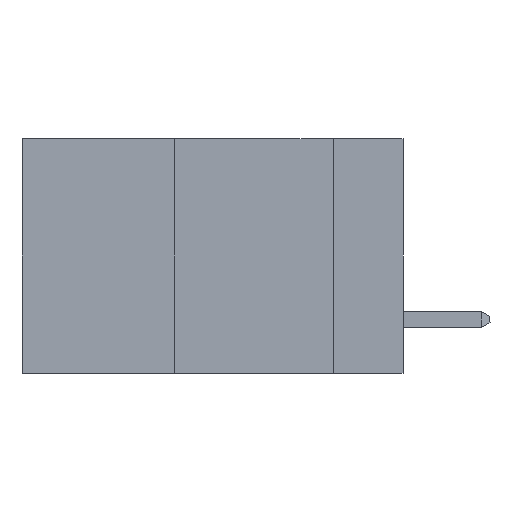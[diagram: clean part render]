
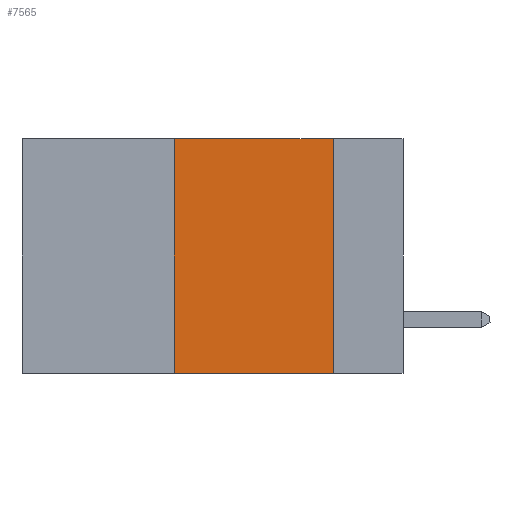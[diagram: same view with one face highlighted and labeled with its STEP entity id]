
A CAD part, left-side view. The second image highlights one B-rep face of the part: STEP entity #7565.
In plain terms, the highlighted planar face has unit normal (-1, 0, 0).
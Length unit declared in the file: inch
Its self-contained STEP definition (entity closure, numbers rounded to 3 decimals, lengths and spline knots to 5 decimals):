
#981 = VECTOR ( 'NONE', #9468, 39.37008 ) ;
#1636 = CARTESIAN_POINT ( 'NONE',  ( 0., 0.6, -0.37 ) ) ;
#1899 = CARTESIAN_POINT ( 'NONE',  ( 0., 0.36, 0. ) ) ;
#2527 = ORIENTED_EDGE ( 'NONE', *, *, #8958, .F. ) ;
#2906 = ORIENTED_EDGE ( 'NONE', *, *, #12449, .T. ) ;
#2966 = VECTOR ( 'NONE', #4611, 39.37008 ) ;
#3118 = DIRECTION ( 'NONE',  ( 0., 0., 1. ) ) ;
#3429 = LINE ( 'NONE', #1636, #981 ) ;
#3470 = CARTESIAN_POINT ( 'NONE',  ( 0., 0.6, 0. ) ) ;
#3562 = VECTOR ( 'NONE', #9497, 39.37008 ) ;
#3888 = CARTESIAN_POINT ( 'NONE',  ( 0., 0.11, 0. ) ) ;
#4048 = EDGE_CURVE ( 'NONE', #14142, #12676, #5926, .T. ) ;
#4592 = DIRECTION ( 'NONE',  ( 0., 0., -1. ) ) ;
#4611 = DIRECTION ( 'NONE',  ( 0., 0., -1. ) ) ;
#5926 = LINE ( 'NONE', #12236, #2966 ) ;
#7234 = LINE ( 'NONE', #9724, #10113 ) ;
#7475 = EDGE_LOOP ( 'NONE', ( #13849, #2527, #14164, #2906 ) ) ;
#7565 = ADVANCED_FACE ( 'NONE', ( #10115 ), #13234, .F. ) ;
#8765 = CARTESIAN_POINT ( 'NONE',  ( 0., 0.36, -0.37 ) ) ;
#8775 = CARTESIAN_POINT ( 'NONE',  ( 0., 0.11, -0.37 ) ) ;
#8958 = EDGE_CURVE ( 'NONE', #10308, #14142, #9435, .T. ) ;
#9435 = LINE ( 'NONE', #12687, #3562 ) ;
#9468 = DIRECTION ( 'NONE',  ( 0., -1., 0. ) ) ;
#9497 = DIRECTION ( 'NONE',  ( 0., -1., 0. ) ) ;
#9724 = CARTESIAN_POINT ( 'NONE',  ( 0., 0.36, 0. ) ) ;
#10113 = VECTOR ( 'NONE', #3118, 39.37008 ) ;
#10115 = FACE_OUTER_BOUND ( 'NONE', #7475, .T. ) ;
#10308 = VERTEX_POINT ( 'NONE', #1899 ) ;
#11118 = DIRECTION ( 'NONE',  ( 1., 0., 0. ) ) ;
#12236 = CARTESIAN_POINT ( 'NONE',  ( 0., 0.11, 0. ) ) ;
#12449 = EDGE_CURVE ( 'NONE', #13183, #12676, #3429, .T. ) ;
#12577 = EDGE_CURVE ( 'NONE', #13183, #10308, #7234, .T. ) ;
#12676 = VERTEX_POINT ( 'NONE', #8775 ) ;
#12687 = CARTESIAN_POINT ( 'NONE',  ( 0., 0.6, 0. ) ) ;
#13183 = VERTEX_POINT ( 'NONE', #8765 ) ;
#13234 = PLANE ( 'NONE',  #13248 ) ;
#13248 = AXIS2_PLACEMENT_3D ( 'NONE', #3470, #11118, #4592 ) ;
#13849 = ORIENTED_EDGE ( 'NONE', *, *, #4048, .F. ) ;
#14142 = VERTEX_POINT ( 'NONE', #3888 ) ;
#14164 = ORIENTED_EDGE ( 'NONE', *, *, #12577, .F. ) ;
